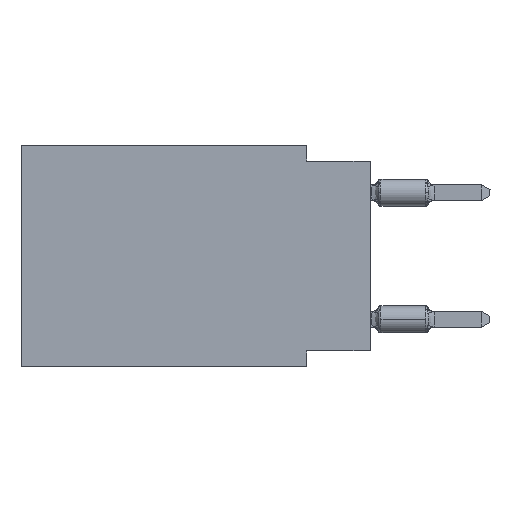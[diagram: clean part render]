
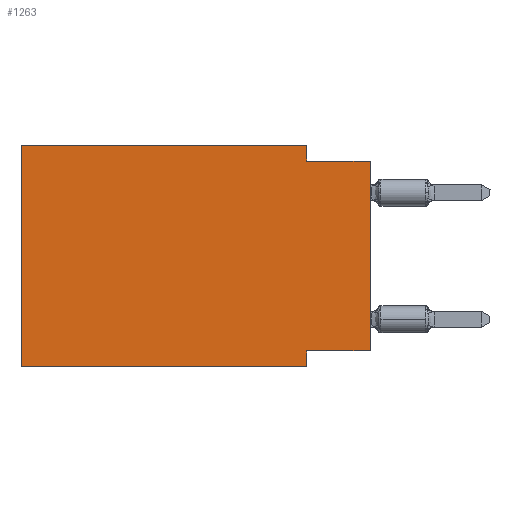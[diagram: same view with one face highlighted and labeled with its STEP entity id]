
A CAD part, left-side view. The second image highlights one B-rep face of the part: STEP entity #1263.
In plain terms, the highlighted planar face has unit normal (-1, 0, 0).
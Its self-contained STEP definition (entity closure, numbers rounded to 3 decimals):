
#232 = LINE ( 'NONE', #22538, #5322 ) ;
#376 = CARTESIAN_POINT ( 'NONE',  ( 0., 13.97, 0. ) ) ;
#1234 = VERTEX_POINT ( 'NONE', #14026 ) ;
#1263 = ADVANCED_FACE ( 'NONE', ( #23964 ), #19498, .F. ) ;
#1305 = ORIENTED_EDGE ( 'NONE', *, *, #25439, .F. ) ;
#1462 = VECTOR ( 'NONE', #28274, 1000. ) ;
#1983 = ORIENTED_EDGE ( 'NONE', *, *, #4177, .F. ) ;
#3173 = DIRECTION ( 'NONE',  ( 1., 0., 0. ) ) ;
#3188 = CARTESIAN_POINT ( 'NONE',  ( 0., 13.97, 0. ) ) ;
#3599 = DIRECTION ( 'NONE',  ( 0., 1., 0. ) ) ;
#3600 = VERTEX_POINT ( 'NONE', #5300 ) ;
#3706 = VECTOR ( 'NONE', #27849, 1000. ) ;
#4177 = EDGE_CURVE ( 'NONE', #26573, #4480, #28534, .T. ) ;
#4235 = CARTESIAN_POINT ( 'NONE',  ( 0., 0., 0. ) ) ;
#4480 = VERTEX_POINT ( 'NONE', #25531 ) ;
#4497 = ORIENTED_EDGE ( 'NONE', *, *, #20736, .F. ) ;
#5050 = VECTOR ( 'NONE', #14877, 1000. ) ;
#5300 = CARTESIAN_POINT ( 'NONE',  ( 0., 0., -8.255 ) ) ;
#5322 = VECTOR ( 'NONE', #24897, 1000. ) ;
#5694 = AXIS2_PLACEMENT_3D ( 'NONE', #10005, #3173, #21293 ) ;
#6404 = EDGE_CURVE ( 'NONE', #19308, #19674, #19075, .T. ) ;
#7036 = CARTESIAN_POINT ( 'NONE',  ( 0., 2.54, 0. ) ) ;
#7061 = VECTOR ( 'NONE', #18929, 1000. ) ;
#8031 = LINE ( 'NONE', #7036, #5050 ) ;
#10005 = CARTESIAN_POINT ( 'NONE',  ( 0., 13.97, 0. ) ) ;
#11456 = CARTESIAN_POINT ( 'NONE',  ( 0., 13.97, -8.89 ) ) ;
#13329 = VECTOR ( 'NONE', #24510, 1000. ) ;
#14026 = CARTESIAN_POINT ( 'NONE',  ( 0., 2.54, -8.255 ) ) ;
#14237 = ORIENTED_EDGE ( 'NONE', *, *, #23778, .T. ) ;
#14280 = ORIENTED_EDGE ( 'NONE', *, *, #28654, .F. ) ;
#14780 = VECTOR ( 'NONE', #22355, 1000. ) ;
#14877 = DIRECTION ( 'NONE',  ( 0., 0., -1. ) ) ;
#14897 = LINE ( 'NONE', #23950, #21963 ) ;
#15896 = EDGE_CURVE ( 'NONE', #3600, #1234, #14897, .T. ) ;
#16234 = EDGE_LOOP ( 'NONE', ( #24455, #1983, #4497, #14280, #21880, #14237, #1305, #17744 ) ) ;
#17320 = LINE ( 'NONE', #4235, #14780 ) ;
#17744 = ORIENTED_EDGE ( 'NONE', *, *, #15896, .F. ) ;
#18369 = CARTESIAN_POINT ( 'NONE',  ( 0., 2.54, 0. ) ) ;
#18787 = LINE ( 'NONE', #376, #3706 ) ;
#18929 = DIRECTION ( 'NONE',  ( 0., 0., 1. ) ) ;
#19075 = LINE ( 'NONE', #3188, #7061 ) ;
#19308 = VERTEX_POINT ( 'NONE', #11456 ) ;
#19498 = PLANE ( 'NONE',  #5694 ) ;
#19511 = VERTEX_POINT ( 'NONE', #27789 ) ;
#19674 = VERTEX_POINT ( 'NONE', #24213 ) ;
#20736 = EDGE_CURVE ( 'NONE', #23894, #26573, #8031, .T. ) ;
#21293 = DIRECTION ( 'NONE',  ( 0., 0., -1. ) ) ;
#21880 = ORIENTED_EDGE ( 'NONE', *, *, #6404, .F. ) ;
#21963 = VECTOR ( 'NONE', #3599, 1000. ) ;
#21994 = CARTESIAN_POINT ( 'NONE',  ( 0., 0., -0.635 ) ) ;
#22355 = DIRECTION ( 'NONE',  ( 0., 0., 1. ) ) ;
#22512 = CARTESIAN_POINT ( 'NONE',  ( 0., 2.54, -0.635 ) ) ;
#22538 = CARTESIAN_POINT ( 'NONE',  ( 0., 13.97, -8.89 ) ) ;
#23778 = EDGE_CURVE ( 'NONE', #19308, #19511, #232, .T. ) ;
#23894 = VERTEX_POINT ( 'NONE', #18369 ) ;
#23950 = CARTESIAN_POINT ( 'NONE',  ( 0., 0., -8.255 ) ) ;
#23964 = FACE_OUTER_BOUND ( 'NONE', #16234, .T. ) ;
#24213 = CARTESIAN_POINT ( 'NONE',  ( 0., 13.97, 0. ) ) ;
#24455 = ORIENTED_EDGE ( 'NONE', *, *, #25224, .T. ) ;
#24510 = DIRECTION ( 'NONE',  ( 0., -1., 0. ) ) ;
#24897 = DIRECTION ( 'NONE',  ( 0., -1., 0. ) ) ;
#25224 = EDGE_CURVE ( 'NONE', #3600, #4480, #17320, .T. ) ;
#25439 = EDGE_CURVE ( 'NONE', #1234, #19511, #27828, .T. ) ;
#25531 = CARTESIAN_POINT ( 'NONE',  ( 0., 0., -0.635 ) ) ;
#26573 = VERTEX_POINT ( 'NONE', #22512 ) ;
#27789 = CARTESIAN_POINT ( 'NONE',  ( 0., 2.54, -8.89 ) ) ;
#27828 = LINE ( 'NONE', #28125, #1462 ) ;
#27849 = DIRECTION ( 'NONE',  ( 0., -1., 0. ) ) ;
#28125 = CARTESIAN_POINT ( 'NONE',  ( 0., 2.54, -8.89 ) ) ;
#28274 = DIRECTION ( 'NONE',  ( 0., 0., -1. ) ) ;
#28534 = LINE ( 'NONE', #21994, #13329 ) ;
#28654 = EDGE_CURVE ( 'NONE', #19674, #23894, #18787, .T. ) ;
